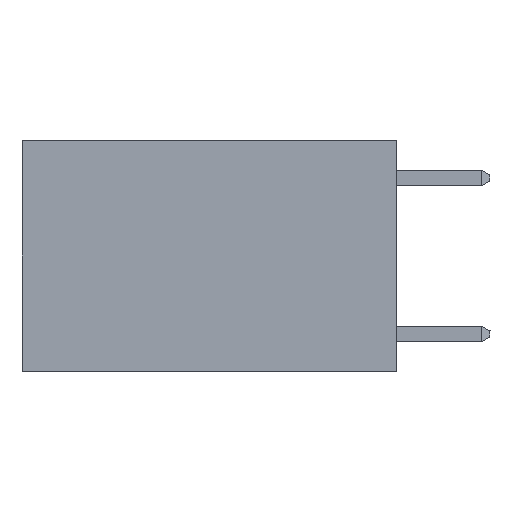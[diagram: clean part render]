
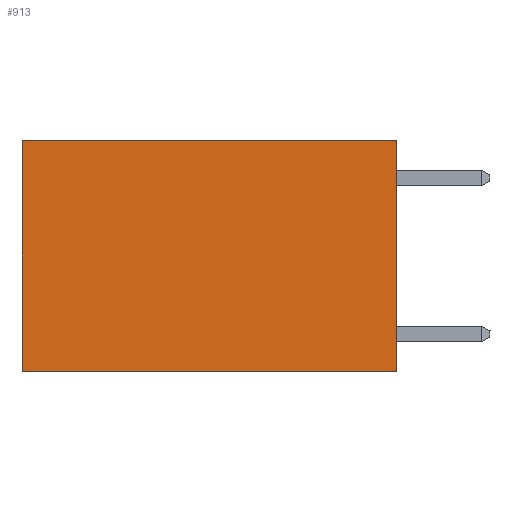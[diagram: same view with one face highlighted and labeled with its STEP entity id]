
A CAD part, left-side view. The second image highlights one B-rep face of the part: STEP entity #913.
In plain terms, the highlighted planar face has unit normal (-1, 0, 0).
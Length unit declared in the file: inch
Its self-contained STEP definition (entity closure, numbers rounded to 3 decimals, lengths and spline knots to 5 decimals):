
#259 = VERTEX_POINT ( 'NONE', #3635 ) ;
#286 = CARTESIAN_POINT ( 'NONE',  ( 0.2625, 0., 0. ) ) ;
#913 = ADVANCED_FACE ( 'NONE', ( #8604 ), #7851, .F. ) ;
#1303 = DIRECTION ( 'NONE',  ( 1., 0., 0. ) ) ;
#1701 = LINE ( 'NONE', #3224, #6912 ) ;
#1918 = ORIENTED_EDGE ( 'NONE', *, *, #7830, .F. ) ;
#1970 = DIRECTION ( 'NONE',  ( 0., 0., -1. ) ) ;
#2163 = LINE ( 'NONE', #4476, #3719 ) ;
#2247 = EDGE_LOOP ( 'NONE', ( #5258, #7096, #1918, #7298 ) ) ;
#2527 = EDGE_CURVE ( 'NONE', #7489, #6494, #1701, .T. ) ;
#2600 = AXIS2_PLACEMENT_3D ( 'NONE', #6998, #1303, #1970 ) ;
#2991 = LINE ( 'NONE', #7669, #6473 ) ;
#3159 = DIRECTION ( 'NONE',  ( 0., 0., -1. ) ) ;
#3224 = CARTESIAN_POINT ( 'NONE',  ( 0.2625, 0., 0. ) ) ;
#3540 = CARTESIAN_POINT ( 'NONE',  ( 0.2625, 0., -0.37 ) ) ;
#3635 = CARTESIAN_POINT ( 'NONE',  ( 0.2625, 0.6, -0.37 ) ) ;
#3719 = VECTOR ( 'NONE', #4502, 39.37008 ) ;
#3745 = CARTESIAN_POINT ( 'NONE',  ( 0.2625, 0., 0. ) ) ;
#4248 = VECTOR ( 'NONE', #3159, 39.37008 ) ;
#4476 = CARTESIAN_POINT ( 'NONE',  ( 0.2625, 0.6, 0. ) ) ;
#4502 = DIRECTION ( 'NONE',  ( 0., 0., -1. ) ) ;
#5258 = ORIENTED_EDGE ( 'NONE', *, *, #6558, .T. ) ;
#5857 = CARTESIAN_POINT ( 'NONE',  ( 0.2625, 0.6, 0. ) ) ;
#5891 = EDGE_CURVE ( 'NONE', #8549, #259, #2991, .T. ) ;
#5999 = DIRECTION ( 'NONE',  ( 0., 1., 0. ) ) ;
#6473 = VECTOR ( 'NONE', #8281, 39.37008 ) ;
#6494 = VERTEX_POINT ( 'NONE', #5857 ) ;
#6558 = EDGE_CURVE ( 'NONE', #6494, #259, #2163, .T. ) ;
#6912 = VECTOR ( 'NONE', #5999, 39.37008 ) ;
#6998 = CARTESIAN_POINT ( 'NONE',  ( 0.2625, 0., 0. ) ) ;
#7096 = ORIENTED_EDGE ( 'NONE', *, *, #5891, .F. ) ;
#7298 = ORIENTED_EDGE ( 'NONE', *, *, #2527, .T. ) ;
#7489 = VERTEX_POINT ( 'NONE', #3745 ) ;
#7669 = CARTESIAN_POINT ( 'NONE',  ( 0.2625, 0., -0.37 ) ) ;
#7818 = LINE ( 'NONE', #286, #4248 ) ;
#7830 = EDGE_CURVE ( 'NONE', #7489, #8549, #7818, .T. ) ;
#7851 = PLANE ( 'NONE',  #2600 ) ;
#8281 = DIRECTION ( 'NONE',  ( 0., 1., 0. ) ) ;
#8549 = VERTEX_POINT ( 'NONE', #3540 ) ;
#8604 = FACE_OUTER_BOUND ( 'NONE', #2247, .T. ) ;
